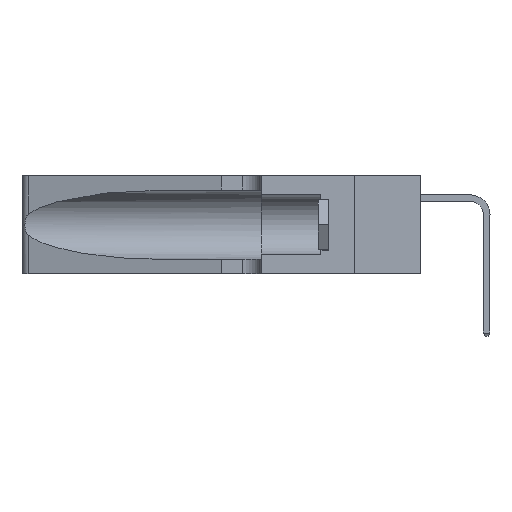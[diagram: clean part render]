
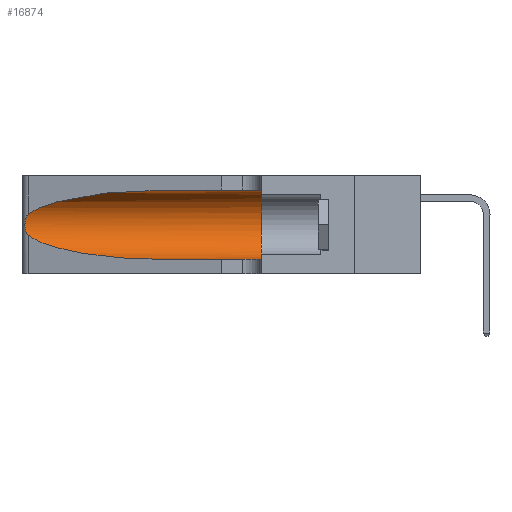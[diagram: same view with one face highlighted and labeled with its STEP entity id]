
A CAD part, left-side view. The second image highlights one B-rep face of the part: STEP entity #16874.
In plain terms, the highlighted cylindrical face has radius 3.308 mm (diameter 6.617 mm), a partial arc.
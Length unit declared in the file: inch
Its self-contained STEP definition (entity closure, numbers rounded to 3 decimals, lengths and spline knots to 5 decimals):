
#268 = ORIENTED_EDGE ( 'NONE', *, *, #25198, .F. ) ;
#886 = EDGE_CURVE ( 'NONE', #9912, #14523, #11976, .T. ) ;
#927 = CARTESIAN_POINT ( 'NONE',  ( 0.1305, 0.35, 0.185 ) ) ;
#1279 = EDGE_CURVE ( 'NONE', #5760, #15398, #13262, .T. ) ;
#1624 = CARTESIAN_POINT ( 'NONE',  ( 0.25787, 1.23484, 0.2124 ) ) ;
#1889 = CYLINDRICAL_SURFACE ( 'NONE', #4398, 0.13025 ) ;
#2009 = DIRECTION ( 'NONE',  ( 0., -1., 0. ) ) ;
#2011 = VERTEX_POINT ( 'NONE', #25604 ) ;
#2096 = ORIENTED_EDGE ( 'NONE', *, *, #29330, .T. ) ;
#3266 = DIRECTION ( 'NONE',  ( 0., 0., 1. ) ) ;
#3957 = CARTESIAN_POINT ( 'NONE',  ( 0.26018, 1.23835, 0.19895 ) ) ;
#4337 = CIRCLE ( 'NONE', #23829, 0.13025 ) ;
#4398 = AXIS2_PLACEMENT_3D ( 'NONE', #6743, #29388, #13385 ) ;
#4607 = VERTEX_POINT ( 'NONE', #7642 ) ;
#5760 = VERTEX_POINT ( 'NONE', #16295 ) ;
#6205 = CARTESIAN_POINT ( 'NONE',  ( 0.25487, 1.22718, 0.22369 ) ) ;
#6311 = CARTESIAN_POINT ( 'NONE',  ( 0.26075, 1.23896, 0.178 ) ) ;
#6743 = CARTESIAN_POINT ( 'NONE',  ( 0.1305, 1.61858, 0.185 ) ) ;
#7390 = EDGE_LOOP ( 'NONE', ( #16928, #18593, #25320, #2096, #268, #23154 ) ) ;
#7534 = EDGE_CURVE ( 'NONE', #9912, #2011, #19547, .T. ) ;
#7629 = CARTESIAN_POINT ( 'NONE',  ( 0.1305, 1.61858, 0.05475 ) ) ;
#7642 = CARTESIAN_POINT ( 'NONE',  ( 0.1305, 0.35, 0.05475 ) ) ;
#8553 = CARTESIAN_POINT ( 'NONE',  ( 0.2373, 1.15595, 0.28018 ) ) ;
#8607 = CARTESIAN_POINT ( 'NONE',  ( 0.25856, 1.23593, 0.16098 ) ) ;
#8700 = CARTESIAN_POINT ( 'NONE',  ( 0.1305, 0.72297, 0.05475 ) ) ;
#8779 = CARTESIAN_POINT ( 'NONE',  ( 0.18966, 0.96281, 0.05475 ) ) ;
#8886 = CARTESIAN_POINT ( 'NONE',  ( 0.25487, 1.22718, 0.14631 ) ) ;
#9719 = CARTESIAN_POINT ( 'NONE',  ( 0.2373, 1.15595, 0.08982 ) ) ;
#9912 = VERTEX_POINT ( 'NONE', #26486 ) ;
#10729 = CARTESIAN_POINT ( 'NONE',  ( 0.1305, 0.72297, 0.05475 ) ) ;
#10915 = CARTESIAN_POINT ( 'NONE',  ( 0.25639, 1.23186, 0.15144 ) ) ;
#11976 =( BOUNDED_CURVE ( )  B_SPLINE_CURVE ( 3, ( #25642, #21795, #8553, #18897 ),
 .UNSPECIFIED., .F., .T. ) 
 B_SPLINE_CURVE_WITH_KNOTS ( ( 4, 4 ),
 ( 1.5708, 2.84003 ),
 .UNSPECIFIED. ) 
 CURVE ( )  GEOMETRIC_REPRESENTATION_ITEM ( )  RATIONAL_B_SPLINE_CURVE ( ( 1., 0.87, 0.87, 1. ) ) 
 REPRESENTATION_ITEM ( '' )  );
#13098 = CARTESIAN_POINT ( 'NONE',  ( 0.25555, 1.22994, 0.2215 ) ) ;
#13198 = CARTESIAN_POINT ( 'NONE',  ( 0.25487, 1.22718, 0.14631 ) ) ;
#13262 =( BOUNDED_CURVE ( )  B_SPLINE_CURVE ( 3, ( #8886, #9719, #8779, #8700 ),
 .UNSPECIFIED., .F., .F. ) 
 B_SPLINE_CURVE_WITH_KNOTS ( ( 4, 4 ),
 ( 3.44316, 4.71239 ),
 .UNSPECIFIED. ) 
 CURVE ( )  GEOMETRIC_REPRESENTATION_ITEM ( )  RATIONAL_B_SPLINE_CURVE ( ( 1., 0.87, 0.87, 1. ) ) 
 REPRESENTATION_ITEM ( '' )  );
#13385 = DIRECTION ( 'NONE',  ( 0., 0., -1. ) ) ;
#14417 = VECTOR ( 'NONE', #21255, 39.37008 ) ;
#14523 = VERTEX_POINT ( 'NONE', #16571 ) ;
#15336 = CARTESIAN_POINT ( 'NONE',  ( 0.25639, 1.23184, 0.21858 ) ) ;
#15398 = VERTEX_POINT ( 'NONE', #10729 ) ;
#16295 = CARTESIAN_POINT ( 'NONE',  ( 0.25487, 1.22718, 0.14631 ) ) ;
#16571 = CARTESIAN_POINT ( 'NONE',  ( 0.25487, 1.22718, 0.22369 ) ) ;
#16874 = ADVANCED_FACE ( 'NONE', ( #20133 ), #1889, .F. ) ;
#16928 = ORIENTED_EDGE ( 'NONE', *, *, #886, .T. ) ;
#16951 = DIRECTION ( 'NONE',  ( 0., 1., 0. ) ) ;
#17616 = CARTESIAN_POINT ( 'NONE',  ( 0.25854, 1.2359, 0.20912 ) ) ;
#17803 = CARTESIAN_POINT ( 'NONE',  ( 0.1305, 1.61858, 0.31525 ) ) ;
#18593 = ORIENTED_EDGE ( 'NONE', *, *, #18748, .T. ) ;
#18748 = EDGE_CURVE ( 'NONE', #14523, #5760, #22962, .T. ) ;
#18897 = CARTESIAN_POINT ( 'NONE',  ( 0.25487, 1.22718, 0.22369 ) ) ;
#19547 = LINE ( 'NONE', #17803, #29402 ) ;
#19938 = CARTESIAN_POINT ( 'NONE',  ( 0.26075, 1.23896, 0.19203 ) ) ;
#20133 = FACE_OUTER_BOUND ( 'NONE', #7390, .T. ) ;
#21255 = DIRECTION ( 'NONE',  ( 0., -1., 0. ) ) ;
#21795 = CARTESIAN_POINT ( 'NONE',  ( 0.18966, 0.96281, 0.31525 ) ) ;
#22219 = CARTESIAN_POINT ( 'NONE',  ( 0.26017, 1.23833, 0.17102 ) ) ;
#22962 = B_SPLINE_CURVE_WITH_KNOTS ( 'NONE', 3,
 ( #6205, #13098, #15336, #1624, #17616, #3957, #19938, #6311, #22219, #8607, #24490, #10915, #26767, #13198 ),
 .UNSPECIFIED., .F., .F.,
 ( 4, 2, 2, 2, 2, 2, 4 ),
 ( 0., 0.00027, 0.00053, 0.00107, 0.0016, 0.00187, 0.00214 ),
 .UNSPECIFIED. ) ;
#23154 = ORIENTED_EDGE ( 'NONE', *, *, #7534, .F. ) ;
#23829 = AXIS2_PLACEMENT_3D ( 'NONE', #927, #16951, #3266 ) ;
#24490 = CARTESIAN_POINT ( 'NONE',  ( 0.25789, 1.23486, 0.15765 ) ) ;
#25198 = EDGE_CURVE ( 'NONE', #2011, #4607, #4337, .T. ) ;
#25320 = ORIENTED_EDGE ( 'NONE', *, *, #1279, .T. ) ;
#25604 = CARTESIAN_POINT ( 'NONE',  ( 0.1305, 0.35, 0.31525 ) ) ;
#25642 = CARTESIAN_POINT ( 'NONE',  ( 0.1305, 0.72297, 0.31525 ) ) ;
#26486 = CARTESIAN_POINT ( 'NONE',  ( 0.1305, 0.72297, 0.31525 ) ) ;
#26767 = CARTESIAN_POINT ( 'NONE',  ( 0.25555, 1.22993, 0.14849 ) ) ;
#27199 = LINE ( 'NONE', #7629, #14417 ) ;
#29330 = EDGE_CURVE ( 'NONE', #15398, #4607, #27199, .T. ) ;
#29388 = DIRECTION ( 'NONE',  ( 0., -1., 0. ) ) ;
#29402 = VECTOR ( 'NONE', #2009, 39.37008 ) ;
